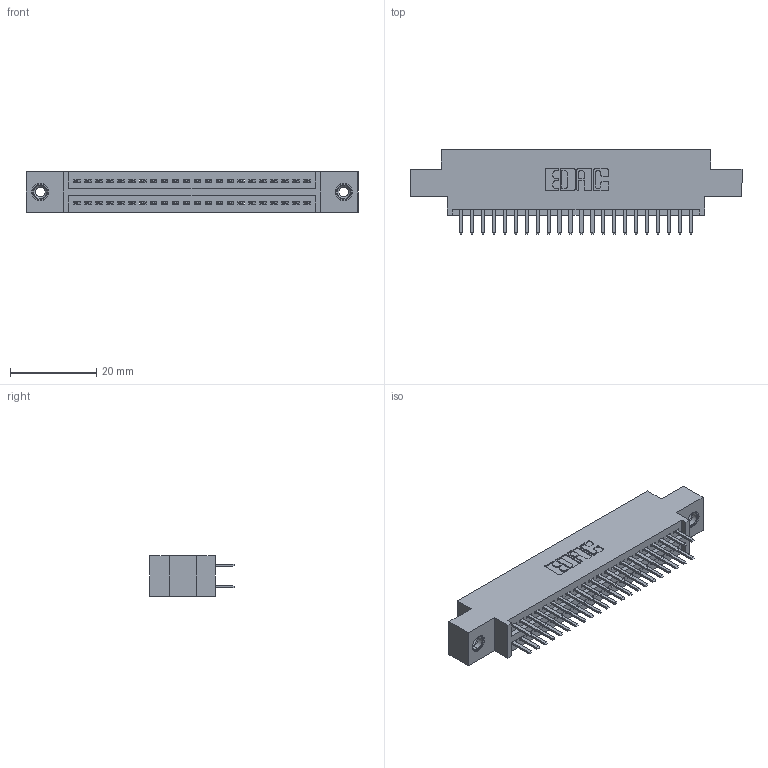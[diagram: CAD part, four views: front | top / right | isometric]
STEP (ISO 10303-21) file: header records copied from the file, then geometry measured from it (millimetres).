
FILE_DESCRIPTION (( 'STEP AP203' ), '1' );
FILE_NAME ('345-044-520-808.STEP', '2018-09-08T09:46:03', ( '' ), ( '' ), 'SwSTEP 2.0', 'SolidWorks 2016', '' );
FILE_SCHEMA (( 'CONFIG_CONTROL_DESIGN' ));
Length unit declared in the file: inch
Products named in the file (4): 345 Part_0.170 Offset - 0.156 Dia-TI; 345-292-001_345-293-120; 345-250-001_345-250-003-102; 345-044-520-808
Assembly tree (47 placements, depth 2):
  345-044-520-808
    345 Part_0.170 Offset - 0.156 Dia-TI
    345-292-001_345-293-120  x44
    345-250-001_345-250-003-102  x2
Bounding box: 77.09 x 19.68 x 9.4 mm (x, y, z)
Volume: 7163.6 mm3; surface area: 10317.4 mm2
Topology: 47 solids, 47 shells, 2566 faces, 7397 edges, 4806 vertices
Faces by surface type: plane 1656, cylinder 894, cone 12, torus 4
Entity records: 21386 total; most frequent: CARTESIAN_POINT 3599, ORIENTED_EDGE 3514, DIRECTION 3211, EDGE_CURVE 1757, LINE 1513, VECTOR 1513, VERTEX_POINT 1164, AXIS2_PLACEMENT_3D 849
